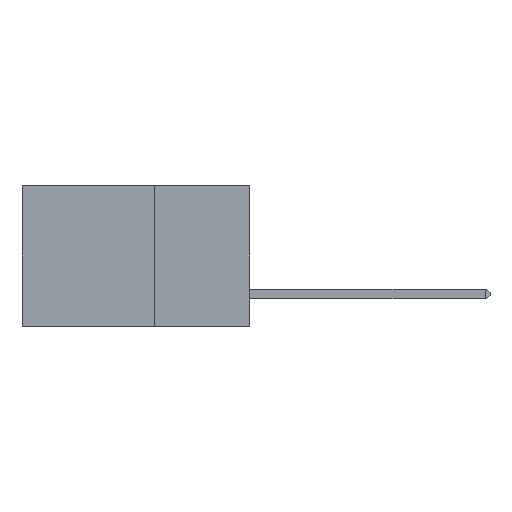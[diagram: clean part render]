
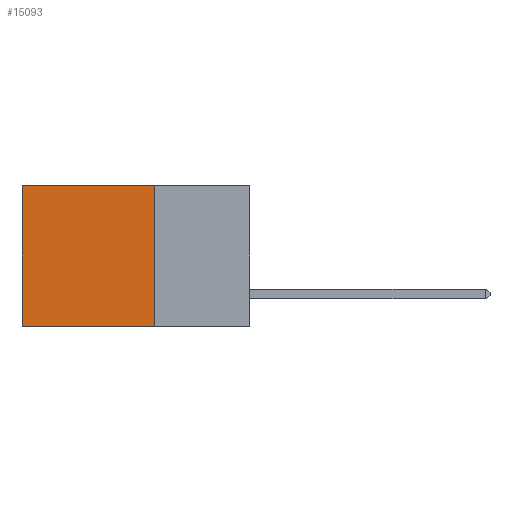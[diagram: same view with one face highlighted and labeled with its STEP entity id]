
A CAD part, left-side view. The second image highlights one B-rep face of the part: STEP entity #15093.
In plain terms, the highlighted planar face has unit normal (-1, 0, 0).
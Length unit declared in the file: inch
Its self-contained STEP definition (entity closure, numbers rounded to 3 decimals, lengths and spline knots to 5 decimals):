
#1229 = EDGE_CURVE ( 'NONE', #14350, #10398, #6681, .T. ) ;
#1564 = VECTOR ( 'NONE', #15148, 39.37008 ) ;
#2854 = CARTESIAN_POINT ( 'NONE',  ( 0.2875, 0.25, 0. ) ) ;
#3164 = EDGE_CURVE ( 'NONE', #4585, #7704, #9080, .T. ) ;
#3716 = PLANE ( 'NONE',  #8461 ) ;
#4019 = CARTESIAN_POINT ( 'NONE',  ( 0.2875, 0.25, 0. ) ) ;
#4585 = VERTEX_POINT ( 'NONE', #11722 ) ;
#5710 = CARTESIAN_POINT ( 'NONE',  ( 0.2875, 0.25, 0. ) ) ;
#6367 = VECTOR ( 'NONE', #15424, 39.37008 ) ;
#6406 = DIRECTION ( 'NONE',  ( 1., 0., 0. ) ) ;
#6530 = ORIENTED_EDGE ( 'NONE', *, *, #8367, .F. ) ;
#6681 = LINE ( 'NONE', #2854, #12674 ) ;
#7555 = EDGE_CURVE ( 'NONE', #14350, #4585, #8507, .T. ) ;
#7704 = VERTEX_POINT ( 'NONE', #10882 ) ;
#8367 = EDGE_CURVE ( 'NONE', #10398, #7704, #15716, .T. ) ;
#8461 = AXIS2_PLACEMENT_3D ( 'NONE', #12403, #6406, #14659 ) ;
#8507 = LINE ( 'NONE', #5710, #1564 ) ;
#8973 = CARTESIAN_POINT ( 'NONE',  ( 0.2875, 0.25, -0.37 ) ) ;
#9080 = LINE ( 'NONE', #10591, #14867 ) ;
#10217 = DIRECTION ( 'NONE',  ( 0., 0., -1. ) ) ;
#10398 = VERTEX_POINT ( 'NONE', #8973 ) ;
#10591 = CARTESIAN_POINT ( 'NONE',  ( 0.2875, 0.6, 0. ) ) ;
#10729 = DIRECTION ( 'NONE',  ( 0., 0., -1. ) ) ;
#10882 = CARTESIAN_POINT ( 'NONE',  ( 0.2875, 0.6, -0.37 ) ) ;
#11722 = CARTESIAN_POINT ( 'NONE',  ( 0.2875, 0.6, 0. ) ) ;
#12403 = CARTESIAN_POINT ( 'NONE',  ( 0.2875, 0.25, 0. ) ) ;
#12674 = VECTOR ( 'NONE', #10729, 39.37008 ) ;
#12894 = ORIENTED_EDGE ( 'NONE', *, *, #1229, .F. ) ;
#12986 = FACE_OUTER_BOUND ( 'NONE', #14330, .T. ) ;
#14311 = CARTESIAN_POINT ( 'NONE',  ( 0.2875, 0.25, -0.37 ) ) ;
#14330 = EDGE_LOOP ( 'NONE', ( #15160, #6530, #12894, #16199 ) ) ;
#14350 = VERTEX_POINT ( 'NONE', #4019 ) ;
#14659 = DIRECTION ( 'NONE',  ( 0., 0., -1. ) ) ;
#14867 = VECTOR ( 'NONE', #10217, 39.37008 ) ;
#15093 = ADVANCED_FACE ( 'NONE', ( #12986 ), #3716, .F. ) ;
#15148 = DIRECTION ( 'NONE',  ( 0., 1., 0. ) ) ;
#15160 = ORIENTED_EDGE ( 'NONE', *, *, #3164, .T. ) ;
#15424 = DIRECTION ( 'NONE',  ( 0., 1., 0. ) ) ;
#15716 = LINE ( 'NONE', #14311, #6367 ) ;
#16199 = ORIENTED_EDGE ( 'NONE', *, *, #7555, .T. ) ;
